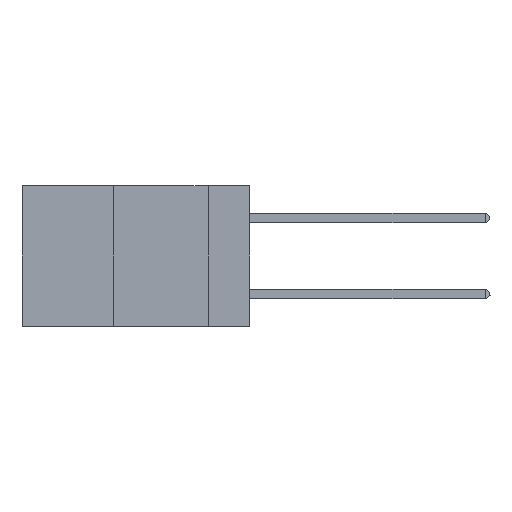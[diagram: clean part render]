
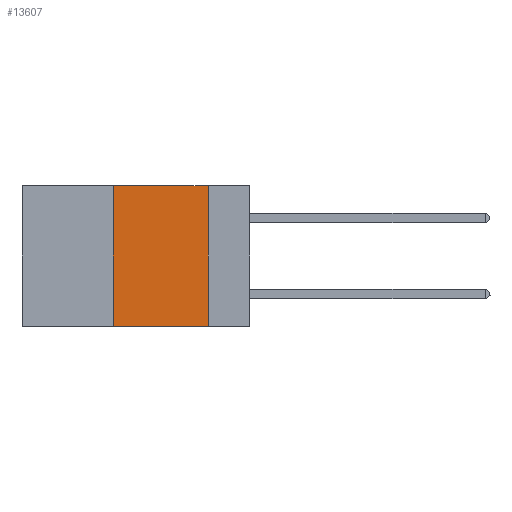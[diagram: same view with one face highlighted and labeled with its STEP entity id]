
A CAD part, left-side view. The second image highlights one B-rep face of the part: STEP entity #13607.
In plain terms, the highlighted planar face has unit normal (-1, 0, 0).
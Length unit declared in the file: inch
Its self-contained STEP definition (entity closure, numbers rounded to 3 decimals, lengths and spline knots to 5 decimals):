
#231 = DIRECTION ( 'NONE',  ( 1., 0., 0. ) ) ;
#564 = VERTEX_POINT ( 'NONE', #24583 ) ;
#690 = CARTESIAN_POINT ( 'NONE',  ( 0., 0.11, -0.37 ) ) ;
#1090 = VECTOR ( 'NONE', #11563, 39.37008 ) ;
#1162 = DIRECTION ( 'NONE',  ( 0., -1., 0. ) ) ;
#2139 = LINE ( 'NONE', #7210, #5466 ) ;
#4479 = VERTEX_POINT ( 'NONE', #21690 ) ;
#4933 = EDGE_CURVE ( 'NONE', #4479, #19946, #2139, .T. ) ;
#5466 = VECTOR ( 'NONE', #14983, 39.37008 ) ;
#7210 = CARTESIAN_POINT ( 'NONE',  ( 0., 0.6, 0. ) ) ;
#7243 = DIRECTION ( 'NONE',  ( 0., 0., -1. ) ) ;
#7719 = ORIENTED_EDGE ( 'NONE', *, *, #25174, .F. ) ;
#9268 = VECTOR ( 'NONE', #1162, 39.37008 ) ;
#10870 = ORIENTED_EDGE ( 'NONE', *, *, #16875, .F. ) ;
#10907 = CARTESIAN_POINT ( 'NONE',  ( 0., 0.6, 0. ) ) ;
#10989 = PLANE ( 'NONE',  #25503 ) ;
#11563 = DIRECTION ( 'NONE',  ( 0., 0., -1. ) ) ;
#12289 = EDGE_CURVE ( 'NONE', #564, #26993, #23717, .T. ) ;
#12408 = CARTESIAN_POINT ( 'NONE',  ( 0., 0.11, 0. ) ) ;
#13597 = ORIENTED_EDGE ( 'NONE', *, *, #4933, .F. ) ;
#13607 = ADVANCED_FACE ( 'NONE', ( #23011 ), #10989, .F. ) ;
#14983 = DIRECTION ( 'NONE',  ( 0., -1., 0. ) ) ;
#16108 = CARTESIAN_POINT ( 'NONE',  ( 0., 0.6, -0.37 ) ) ;
#16668 = ORIENTED_EDGE ( 'NONE', *, *, #12289, .T. ) ;
#16875 = EDGE_CURVE ( 'NONE', #564, #4479, #22133, .T. ) ;
#16890 = LINE ( 'NONE', #19834, #1090 ) ;
#18414 = DIRECTION ( 'NONE',  ( 0., 0., 1. ) ) ;
#19834 = CARTESIAN_POINT ( 'NONE',  ( 0., 0.11, 0. ) ) ;
#19946 = VERTEX_POINT ( 'NONE', #12408 ) ;
#21690 = CARTESIAN_POINT ( 'NONE',  ( 0., 0.36, 0. ) ) ;
#22133 = LINE ( 'NONE', #24885, #24815 ) ;
#23011 = FACE_OUTER_BOUND ( 'NONE', #26965, .T. ) ;
#23717 = LINE ( 'NONE', #16108, #9268 ) ;
#24583 = CARTESIAN_POINT ( 'NONE',  ( 0., 0.36, -0.37 ) ) ;
#24815 = VECTOR ( 'NONE', #18414, 39.37008 ) ;
#24885 = CARTESIAN_POINT ( 'NONE',  ( 0., 0.36, 0. ) ) ;
#25174 = EDGE_CURVE ( 'NONE', #19946, #26993, #16890, .T. ) ;
#25503 = AXIS2_PLACEMENT_3D ( 'NONE', #10907, #231, #7243 ) ;
#26965 = EDGE_LOOP ( 'NONE', ( #7719, #13597, #10870, #16668 ) ) ;
#26993 = VERTEX_POINT ( 'NONE', #690 ) ;
